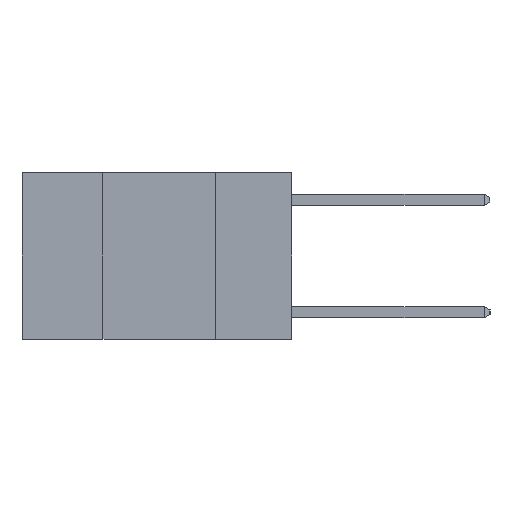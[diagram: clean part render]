
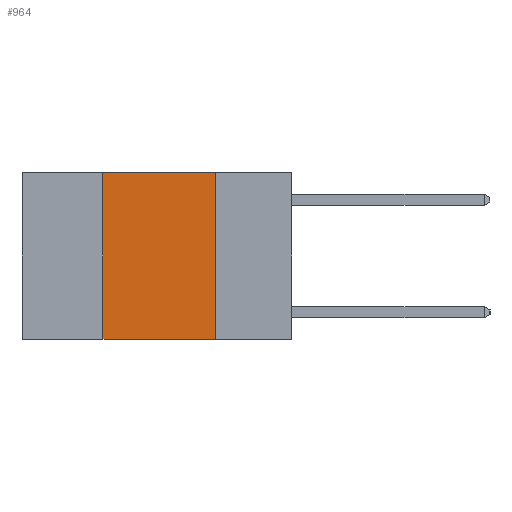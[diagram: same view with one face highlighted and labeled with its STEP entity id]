
A CAD part, left-side view. The second image highlights one B-rep face of the part: STEP entity #964.
In plain terms, the highlighted planar face has unit normal (-1, 0, 0).
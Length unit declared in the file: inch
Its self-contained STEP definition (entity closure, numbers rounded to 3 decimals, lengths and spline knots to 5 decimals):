
#788 = ORIENTED_EDGE ( 'NONE', *, *, #3065, .T. ) ;
#818 = CARTESIAN_POINT ( 'NONE',  ( 0., 0.6, -0.37 ) ) ;
#835 = VERTEX_POINT ( 'NONE', #9145 ) ;
#899 = DIRECTION ( 'NONE',  ( 0., -1., 0. ) ) ;
#964 = ADVANCED_FACE ( 'NONE', ( #9899 ), #3264, .F. ) ;
#1114 = DIRECTION ( 'NONE',  ( 1., 0., 0. ) ) ;
#1457 = VERTEX_POINT ( 'NONE', #3469 ) ;
#1868 = EDGE_CURVE ( 'NONE', #10484, #1457, #8361, .T. ) ;
#2362 = VECTOR ( 'NONE', #9952, 39.37008 ) ;
#2468 = LINE ( 'NONE', #818, #9733 ) ;
#2672 = CARTESIAN_POINT ( 'NONE',  ( 0., 0.42, 0. ) ) ;
#2731 = ORIENTED_EDGE ( 'NONE', *, *, #3945, .F. ) ;
#2776 = AXIS2_PLACEMENT_3D ( 'NONE', #10709, #1114, #6639 ) ;
#3033 = ORIENTED_EDGE ( 'NONE', *, *, #10281, .F. ) ;
#3065 = EDGE_CURVE ( 'NONE', #10878, #835, #2468, .T. ) ;
#3264 = PLANE ( 'NONE',  #2776 ) ;
#3469 = CARTESIAN_POINT ( 'NONE',  ( 0., 0.17, 0. ) ) ;
#3576 = CARTESIAN_POINT ( 'NONE',  ( 0., 0.42, -0.37 ) ) ;
#3641 = LINE ( 'NONE', #2672, #2362 ) ;
#3945 = EDGE_CURVE ( 'NONE', #1457, #835, #7043, .T. ) ;
#4608 = VECTOR ( 'NONE', #5859, 39.37008 ) ;
#5364 = VECTOR ( 'NONE', #899, 39.37008 ) ;
#5859 = DIRECTION ( 'NONE',  ( 0., 0., -1. ) ) ;
#6639 = DIRECTION ( 'NONE',  ( 0., 0., -1. ) ) ;
#7043 = LINE ( 'NONE', #10351, #4608 ) ;
#7306 = DIRECTION ( 'NONE',  ( 0., -1., 0. ) ) ;
#8305 = CARTESIAN_POINT ( 'NONE',  ( 0., 0.6, 0. ) ) ;
#8361 = LINE ( 'NONE', #8305, #5364 ) ;
#8441 = CARTESIAN_POINT ( 'NONE',  ( 0., 0.42, 0. ) ) ;
#9145 = CARTESIAN_POINT ( 'NONE',  ( 0., 0.17, -0.37 ) ) ;
#9321 = EDGE_LOOP ( 'NONE', ( #2731, #9984, #3033, #788 ) ) ;
#9733 = VECTOR ( 'NONE', #7306, 39.37008 ) ;
#9899 = FACE_OUTER_BOUND ( 'NONE', #9321, .T. ) ;
#9952 = DIRECTION ( 'NONE',  ( 0., 0., 1. ) ) ;
#9984 = ORIENTED_EDGE ( 'NONE', *, *, #1868, .F. ) ;
#10281 = EDGE_CURVE ( 'NONE', #10878, #10484, #3641, .T. ) ;
#10351 = CARTESIAN_POINT ( 'NONE',  ( 0., 0.17, 0. ) ) ;
#10484 = VERTEX_POINT ( 'NONE', #8441 ) ;
#10709 = CARTESIAN_POINT ( 'NONE',  ( 0., 0.6, 0. ) ) ;
#10878 = VERTEX_POINT ( 'NONE', #3576 ) ;
